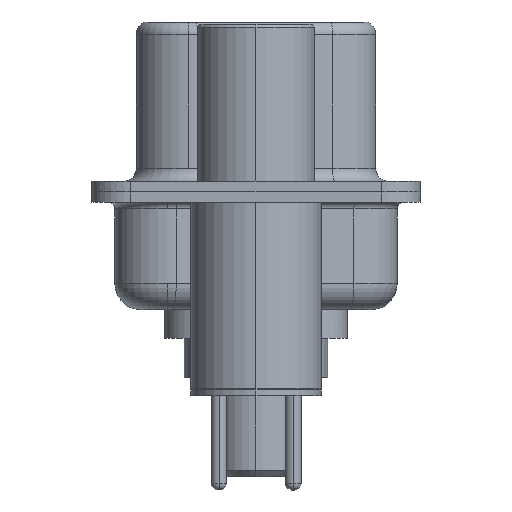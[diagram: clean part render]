
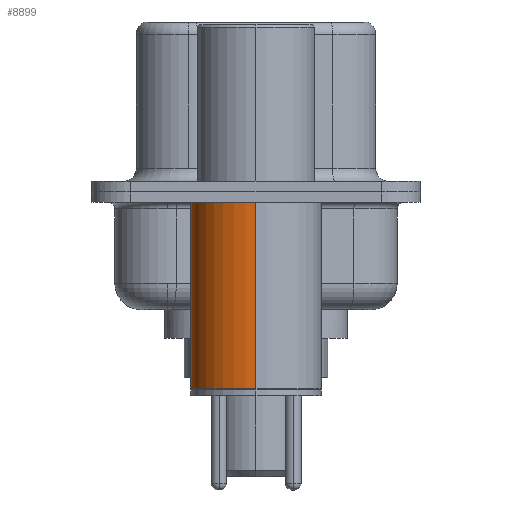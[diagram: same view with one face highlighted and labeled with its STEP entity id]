
A CAD part, left-side view. The second image highlights one B-rep face of the part: STEP entity #8899.
In plain terms, the highlighted cylindrical face has radius 2.5 mm (diameter 5 mm), a partial arc.
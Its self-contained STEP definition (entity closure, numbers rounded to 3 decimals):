
#335 = DIRECTION ( 'NONE',  ( 0., 0., 1. ) ) ;
#1010 = DIRECTION ( 'NONE',  ( 1., 0., 0. ) ) ;
#1026 = ORIENTED_EDGE ( 'NONE', *, *, #2408, .T. ) ;
#1519 = CIRCLE ( 'NONE', #10857, 2.5 ) ;
#1580 = EDGE_LOOP ( 'NONE', ( #9047, #1026, #14009, #22756 ) ) ;
#2381 = DIRECTION ( 'NONE',  ( 0., 0., 1. ) ) ;
#2408 = EDGE_CURVE ( 'NONE', #16654, #6376, #9677, .T. ) ;
#6376 = VERTEX_POINT ( 'NONE', #14079 ) ;
#7195 = CARTESIAN_POINT ( 'NONE',  ( 2.5, 0., -0.4 ) ) ;
#7378 = VERTEX_POINT ( 'NONE', #14562 ) ;
#7907 = CARTESIAN_POINT ( 'NONE',  ( 0., 0., 0.581 ) ) ;
#8319 = CARTESIAN_POINT ( 'NONE',  ( -2.5, 0., -7.525 ) ) ;
#8899 = ADVANCED_FACE ( 'NONE', ( #19559 ), #23796, .T. ) ;
#9047 = ORIENTED_EDGE ( 'NONE', *, *, #11734, .T. ) ;
#9659 = VECTOR ( 'NONE', #15930, 1000. ) ;
#9677 = LINE ( 'NONE', #18747, #18975 ) ;
#10857 = AXIS2_PLACEMENT_3D ( 'NONE', #11657, #335, #13554 ) ;
#11657 = CARTESIAN_POINT ( 'NONE',  ( 0., 0., -0.4 ) ) ;
#11734 = EDGE_CURVE ( 'NONE', #7378, #16654, #21715, .T. ) ;
#12224 = AXIS2_PLACEMENT_3D ( 'NONE', #7907, #2381, #13669 ) ;
#12236 = EDGE_CURVE ( 'NONE', #22721, #6376, #1519, .T. ) ;
#12324 = DIRECTION ( 'NONE',  ( 0., 0., 1. ) ) ;
#13554 = DIRECTION ( 'NONE',  ( 1., 0., 0. ) ) ;
#13669 = DIRECTION ( 'NONE',  ( 1., 0., 0. ) ) ;
#14009 = ORIENTED_EDGE ( 'NONE', *, *, #12236, .F. ) ;
#14074 = CARTESIAN_POINT ( 'NONE',  ( 2.5, 0., 0.581 ) ) ;
#14079 = CARTESIAN_POINT ( 'NONE',  ( -2.5, 0., -0.4 ) ) ;
#14562 = CARTESIAN_POINT ( 'NONE',  ( 2.5, 0., -7.525 ) ) ;
#15930 = DIRECTION ( 'NONE',  ( 0., 0., 1. ) ) ;
#16654 = VERTEX_POINT ( 'NONE', #8319 ) ;
#17114 = EDGE_CURVE ( 'NONE', #7378, #22721, #19549, .T. ) ;
#18747 = CARTESIAN_POINT ( 'NONE',  ( -2.5, 0., 0.581 ) ) ;
#18975 = VECTOR ( 'NONE', #23184, 1000. ) ;
#19549 = LINE ( 'NONE', #14074, #9659 ) ;
#19559 = FACE_OUTER_BOUND ( 'NONE', #1580, .T. ) ;
#20471 = AXIS2_PLACEMENT_3D ( 'NONE', #23332, #12324, #1010 ) ;
#21715 = CIRCLE ( 'NONE', #20471, 2.5 ) ;
#22721 = VERTEX_POINT ( 'NONE', #7195 ) ;
#22756 = ORIENTED_EDGE ( 'NONE', *, *, #17114, .F. ) ;
#23184 = DIRECTION ( 'NONE',  ( 0., 0., 1. ) ) ;
#23332 = CARTESIAN_POINT ( 'NONE',  ( 0., 0., -7.525 ) ) ;
#23796 = CYLINDRICAL_SURFACE ( 'NONE', #12224, 2.5 ) ;
